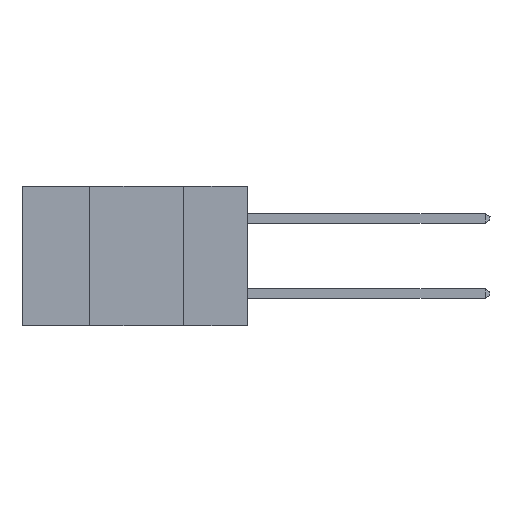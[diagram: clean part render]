
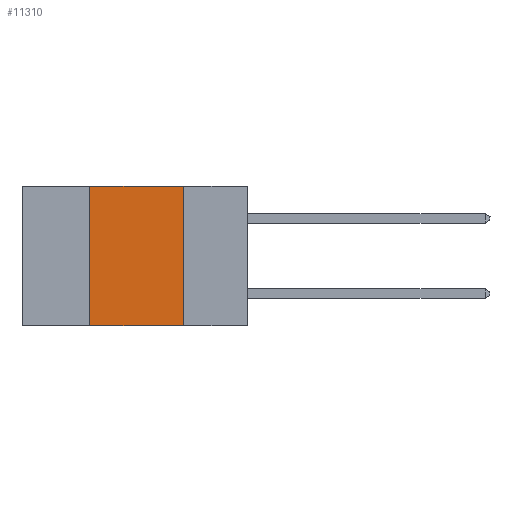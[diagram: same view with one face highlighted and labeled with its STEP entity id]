
A CAD part, left-side view. The second image highlights one B-rep face of the part: STEP entity #11310.
In plain terms, the highlighted planar face has unit normal (-1, 0, 0).
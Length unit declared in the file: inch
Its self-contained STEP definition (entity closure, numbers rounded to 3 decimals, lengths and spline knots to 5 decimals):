
#184 = VERTEX_POINT ( 'NONE', #2091 ) ;
#786 = CARTESIAN_POINT ( 'NONE',  ( 0., 0.17, 0. ) ) ;
#1036 = VERTEX_POINT ( 'NONE', #786 ) ;
#1754 = AXIS2_PLACEMENT_3D ( 'NONE', #7424, #14896, #10555 ) ;
#2091 = CARTESIAN_POINT ( 'NONE',  ( 0., 0.42, 0. ) ) ;
#2150 = DIRECTION ( 'NONE',  ( 0., 0., -1. ) ) ;
#2466 = DIRECTION ( 'NONE',  ( 0., 0., 1. ) ) ;
#3061 = EDGE_CURVE ( 'NONE', #18114, #184, #18298, .T. ) ;
#3175 = ORIENTED_EDGE ( 'NONE', *, *, #10683, .F. ) ;
#3689 = LINE ( 'NONE', #10945, #8985 ) ;
#4442 = ORIENTED_EDGE ( 'NONE', *, *, #5563, .F. ) ;
#4998 = DIRECTION ( 'NONE',  ( 0., -1., 0. ) ) ;
#5563 = EDGE_CURVE ( 'NONE', #1036, #5920, #13656, .T. ) ;
#5920 = VERTEX_POINT ( 'NONE', #7288 ) ;
#6740 = LINE ( 'NONE', #9679, #11674 ) ;
#7288 = CARTESIAN_POINT ( 'NONE',  ( 0., 0.17, -0.37 ) ) ;
#7424 = CARTESIAN_POINT ( 'NONE',  ( 0., 0.6, 0. ) ) ;
#7805 = CARTESIAN_POINT ( 'NONE',  ( 0., 0.42, -0.37 ) ) ;
#8486 = CARTESIAN_POINT ( 'NONE',  ( 0., 0.42, -0.37 ) ) ;
#8985 = VECTOR ( 'NONE', #4998, 39.37008 ) ;
#9134 = FACE_OUTER_BOUND ( 'NONE', #15123, .T. ) ;
#9258 = ORIENTED_EDGE ( 'NONE', *, *, #3061, .F. ) ;
#9481 = CARTESIAN_POINT ( 'NONE',  ( 0., 0.17, -0.37 ) ) ;
#9596 = EDGE_CURVE ( 'NONE', #18114, #5920, #3689, .T. ) ;
#9679 = CARTESIAN_POINT ( 'NONE',  ( 0., 0.6, 0. ) ) ;
#10010 = VECTOR ( 'NONE', #2466, 39.37008 ) ;
#10555 = DIRECTION ( 'NONE',  ( 0., 0., -1. ) ) ;
#10683 = EDGE_CURVE ( 'NONE', #184, #1036, #6740, .T. ) ;
#10945 = CARTESIAN_POINT ( 'NONE',  ( 0., 0.6, -0.37 ) ) ;
#11310 = ADVANCED_FACE ( 'NONE', ( #9134 ), #11877, .F. ) ;
#11674 = VECTOR ( 'NONE', #18448, 39.37008 ) ;
#11877 = PLANE ( 'NONE',  #1754 ) ;
#13134 = VECTOR ( 'NONE', #2150, 39.37008 ) ;
#13656 = LINE ( 'NONE', #9481, #13134 ) ;
#13875 = ORIENTED_EDGE ( 'NONE', *, *, #9596, .T. ) ;
#14896 = DIRECTION ( 'NONE',  ( 1., 0., 0. ) ) ;
#15123 = EDGE_LOOP ( 'NONE', ( #4442, #3175, #9258, #13875 ) ) ;
#18114 = VERTEX_POINT ( 'NONE', #7805 ) ;
#18298 = LINE ( 'NONE', #8486, #10010 ) ;
#18448 = DIRECTION ( 'NONE',  ( 0., -1., 0. ) ) ;
